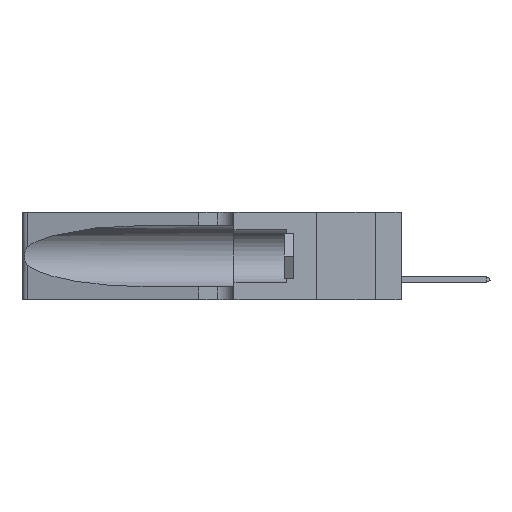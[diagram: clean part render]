
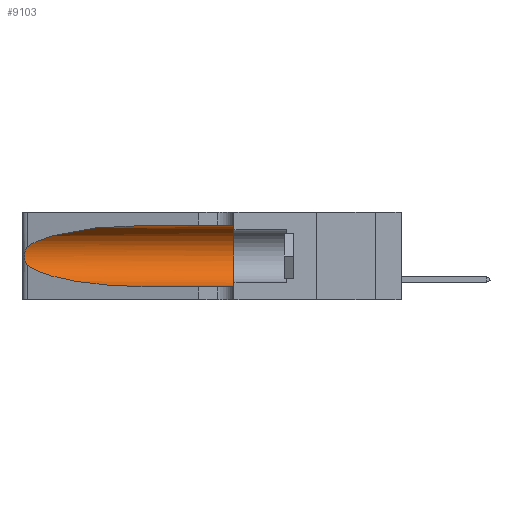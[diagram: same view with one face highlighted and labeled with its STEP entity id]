
A CAD part, left-side view. The second image highlights one B-rep face of the part: STEP entity #9103.
In plain terms, the highlighted cylindrical face has radius 3.308 mm (diameter 6.617 mm), a partial arc.
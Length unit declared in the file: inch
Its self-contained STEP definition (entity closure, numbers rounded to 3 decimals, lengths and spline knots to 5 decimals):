
#329 = CARTESIAN_POINT ( 'NONE',  ( 0.25789, 1.23486, 0.15765 ) ) ;
#547 = CARTESIAN_POINT ( 'NONE',  ( 0.25787, 1.23484, 0.2124 ) ) ;
#838 = LINE ( 'NONE', #32517, #12274 ) ;
#1820 = CARTESIAN_POINT ( 'NONE',  ( 0.26017, 1.23833, 0.17102 ) ) ;
#1883 = ORIENTED_EDGE ( 'NONE', *, *, #15156, .F. ) ;
#1954 = CARTESIAN_POINT ( 'NONE',  ( 0.25487, 1.22718, 0.22369 ) ) ;
#1980 =( BOUNDED_CURVE ( )  B_SPLINE_CURVE ( 3, ( #19099, #31404, #2954, #1954 ),
 .UNSPECIFIED., .F., .T. ) 
 B_SPLINE_CURVE_WITH_KNOTS ( ( 4, 4 ),
 ( 1.5708, 2.84003 ),
 .UNSPECIFIED. ) 
 CURVE ( )  GEOMETRIC_REPRESENTATION_ITEM ( )  RATIONAL_B_SPLINE_CURVE ( ( 1., 0.87, 0.87, 1. ) ) 
 REPRESENTATION_ITEM ( '' )  );
#2149 = CARTESIAN_POINT ( 'NONE',  ( 0.1305, 0.72297, 0.31525 ) ) ;
#2413 = CARTESIAN_POINT ( 'NONE',  ( 0.1305, 0.72297, 0.05475 ) ) ;
#2511 = LINE ( 'NONE', #5457, #34540 ) ;
#2954 = CARTESIAN_POINT ( 'NONE',  ( 0.2373, 1.15595, 0.28018 ) ) ;
#3993 = CIRCLE ( 'NONE', #17398, 0.13025 ) ;
#5457 = CARTESIAN_POINT ( 'NONE',  ( 0.1305, 1.61858, 0.05475 ) ) ;
#5863 = CARTESIAN_POINT ( 'NONE',  ( 0.1305, 0.35, 0.31525 ) ) ;
#5995 = CARTESIAN_POINT ( 'NONE',  ( 0.25555, 1.22993, 0.14849 ) ) ;
#6571 = DIRECTION ( 'NONE',  ( 0., 0., -1. ) ) ;
#8563 = AXIS2_PLACEMENT_3D ( 'NONE', #18157, #21090, #6571 ) ;
#8781 = ORIENTED_EDGE ( 'NONE', *, *, #15241, .T. ) ;
#9037 = CYLINDRICAL_SURFACE ( 'NONE', #8563, 0.13025 ) ;
#9103 = ADVANCED_FACE ( 'NONE', ( #18342 ), #9037, .F. ) ;
#9157 = EDGE_CURVE ( 'NONE', #26499, #32453, #2511, .T. ) ;
#12274 = VECTOR ( 'NONE', #21624, 39.37008 ) ;
#12696 = VERTEX_POINT ( 'NONE', #2149 ) ;
#12885 = ORIENTED_EDGE ( 'NONE', *, *, #9157, .T. ) ;
#13105 = CARTESIAN_POINT ( 'NONE',  ( 0.25487, 1.22718, 0.14631 ) ) ;
#14252 = CARTESIAN_POINT ( 'NONE',  ( 0.25639, 1.23186, 0.15144 ) ) ;
#15156 = EDGE_CURVE ( 'NONE', #26691, #32453, #3993, .T. ) ;
#15241 = EDGE_CURVE ( 'NONE', #12696, #23035, #1980, .T. ) ;
#16964 = ORIENTED_EDGE ( 'NONE', *, *, #32630, .T. ) ;
#17141 = CARTESIAN_POINT ( 'NONE',  ( 0.26018, 1.23835, 0.19895 ) ) ;
#17398 = AXIS2_PLACEMENT_3D ( 'NONE', #31395, #23075, #20773 ) ;
#18157 = CARTESIAN_POINT ( 'NONE',  ( 0.1305, 1.61858, 0.185 ) ) ;
#18342 = FACE_OUTER_BOUND ( 'NONE', #22018, .T. ) ;
#18548 = CARTESIAN_POINT ( 'NONE',  ( 0.26075, 1.23896, 0.19203 ) ) ;
#19099 = CARTESIAN_POINT ( 'NONE',  ( 0.1305, 0.72297, 0.31525 ) ) ;
#19429 = CARTESIAN_POINT ( 'NONE',  ( 0.25487, 1.22718, 0.22369 ) ) ;
#19583 = ORIENTED_EDGE ( 'NONE', *, *, #24249, .T. ) ;
#20773 = DIRECTION ( 'NONE',  ( 0., 0., 1. ) ) ;
#21090 = DIRECTION ( 'NONE',  ( 0., -1., 0. ) ) ;
#21624 = DIRECTION ( 'NONE',  ( 0., -1., 0. ) ) ;
#21717 = CARTESIAN_POINT ( 'NONE',  ( 0.2373, 1.15595, 0.08982 ) ) ;
#22018 = EDGE_LOOP ( 'NONE', ( #8781, #19583, #16964, #12885, #1883, #35699 ) ) ;
#23035 = VERTEX_POINT ( 'NONE', #35657 ) ;
#23075 = DIRECTION ( 'NONE',  ( 0., 1., 0. ) ) ;
#24249 = EDGE_CURVE ( 'NONE', #23035, #28368, #29173, .T. ) ;
#24943 =( BOUNDED_CURVE ( )  B_SPLINE_CURVE ( 3, ( #13105, #21717, #33321, #2413 ),
 .UNSPECIFIED., .F., .T. ) 
 B_SPLINE_CURVE_WITH_KNOTS ( ( 4, 4 ),
 ( 3.44316, 4.71239 ),
 .UNSPECIFIED. ) 
 CURVE ( )  GEOMETRIC_REPRESENTATION_ITEM ( )  RATIONAL_B_SPLINE_CURVE ( ( 1., 0.87, 0.87, 1. ) ) 
 REPRESENTATION_ITEM ( '' )  );
#25149 = DIRECTION ( 'NONE',  ( 0., -1., 0. ) ) ;
#25407 = CARTESIAN_POINT ( 'NONE',  ( 0.25639, 1.23184, 0.21858 ) ) ;
#25668 = CARTESIAN_POINT ( 'NONE',  ( 0.25487, 1.22718, 0.14631 ) ) ;
#26499 = VERTEX_POINT ( 'NONE', #29765 ) ;
#26691 = VERTEX_POINT ( 'NONE', #5863 ) ;
#27861 = CARTESIAN_POINT ( 'NONE',  ( 0.25555, 1.22994, 0.2215 ) ) ;
#28221 = EDGE_CURVE ( 'NONE', #12696, #26691, #838, .T. ) ;
#28368 = VERTEX_POINT ( 'NONE', #29787 ) ;
#28912 = CARTESIAN_POINT ( 'NONE',  ( 0.1305, 0.35, 0.05475 ) ) ;
#29173 = B_SPLINE_CURVE_WITH_KNOTS ( 'NONE', 3,
 ( #19429, #27861, #25407, #547, #31129, #17141, #18548, #31218, #1820, #32601, #329, #14252, #5995, #25668 ),
 .UNSPECIFIED., .F., .F.,
 ( 4, 2, 2, 2, 2, 2, 4 ),
 ( 0., 0.00027, 0.00053, 0.00107, 0.0016, 0.00187, 0.00214 ),
 .UNSPECIFIED. ) ;
#29765 = CARTESIAN_POINT ( 'NONE',  ( 0.1305, 0.72297, 0.05475 ) ) ;
#29787 = CARTESIAN_POINT ( 'NONE',  ( 0.25487, 1.22718, 0.14631 ) ) ;
#31129 = CARTESIAN_POINT ( 'NONE',  ( 0.25854, 1.2359, 0.20912 ) ) ;
#31218 = CARTESIAN_POINT ( 'NONE',  ( 0.26075, 1.23896, 0.178 ) ) ;
#31395 = CARTESIAN_POINT ( 'NONE',  ( 0.1305, 0.35, 0.185 ) ) ;
#31404 = CARTESIAN_POINT ( 'NONE',  ( 0.18966, 0.96281, 0.31525 ) ) ;
#32453 = VERTEX_POINT ( 'NONE', #28912 ) ;
#32517 = CARTESIAN_POINT ( 'NONE',  ( 0.1305, 1.61858, 0.31525 ) ) ;
#32601 = CARTESIAN_POINT ( 'NONE',  ( 0.25856, 1.23593, 0.16098 ) ) ;
#32630 = EDGE_CURVE ( 'NONE', #28368, #26499, #24943, .T. ) ;
#33321 = CARTESIAN_POINT ( 'NONE',  ( 0.18966, 0.96281, 0.05475 ) ) ;
#34540 = VECTOR ( 'NONE', #25149, 39.37008 ) ;
#35657 = CARTESIAN_POINT ( 'NONE',  ( 0.25487, 1.22718, 0.22369 ) ) ;
#35699 = ORIENTED_EDGE ( 'NONE', *, *, #28221, .F. ) ;
